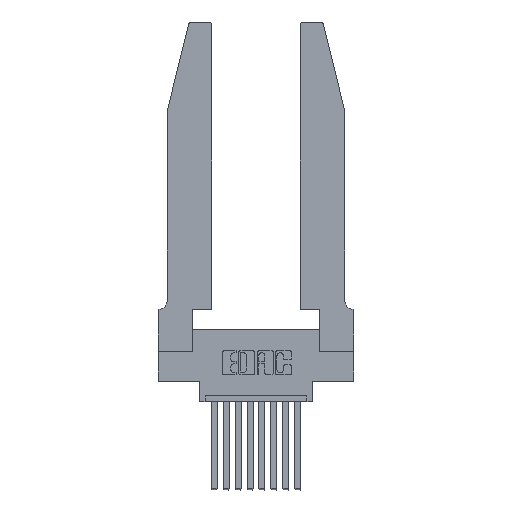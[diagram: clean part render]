
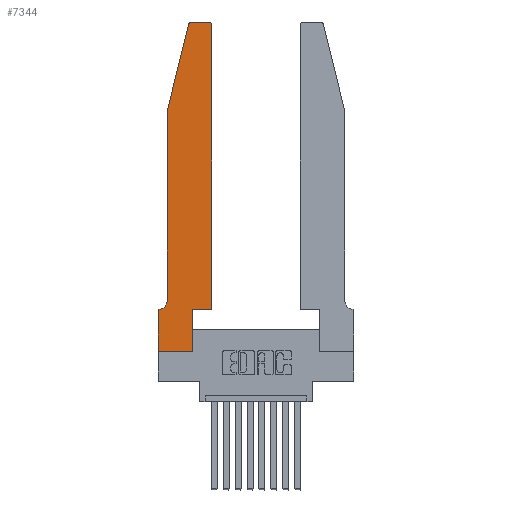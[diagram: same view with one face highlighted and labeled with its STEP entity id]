
A CAD part, top view. The second image highlights one B-rep face of the part: STEP entity #7344.
In plain terms, the highlighted planar face has unit normal (0, 0, 1).
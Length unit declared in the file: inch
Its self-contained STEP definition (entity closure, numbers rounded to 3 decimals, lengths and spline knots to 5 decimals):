
#41 = EDGE_CURVE ( 'NONE', #12247, #8929, #467, .T. ) ;
#159 = CARTESIAN_POINT ( 'NONE',  ( 0.2865, 0.35, 0.37 ) ) ;
#467 = LINE ( 'NONE', #1567, #12608 ) ;
#537 = LINE ( 'NONE', #10434, #8057 ) ;
#677 = DIRECTION ( 'NONE',  ( 0., 0., 1. ) ) ;
#807 = CARTESIAN_POINT ( 'NONE',  ( 0., 0.35, 0.37 ) ) ;
#912 = VERTEX_POINT ( 'NONE', #8366 ) ;
#1132 = VECTOR ( 'NONE', #11473, 39.37008 ) ;
#1176 = VECTOR ( 'NONE', #4415, 39.37008 ) ;
#1204 = LINE ( 'NONE', #14419, #13543 ) ;
#1209 = ORIENTED_EDGE ( 'NONE', *, *, #1664, .T. ) ;
#1481 = ORIENTED_EDGE ( 'NONE', *, *, #13996, .T. ) ;
#1500 = LINE ( 'NONE', #4461, #1132 ) ;
#1567 = CARTESIAN_POINT ( 'NONE',  ( 0.4505, 0.35, 0.37 ) ) ;
#1613 = VERTEX_POINT ( 'NONE', #807 ) ;
#1664 = EDGE_CURVE ( 'NONE', #12188, #10564, #9046, .T. ) ;
#2056 = DIRECTION ( 'NONE',  ( 0., 0., 1. ) ) ;
#2314 = DIRECTION ( 'NONE',  ( 1., 0., 0. ) ) ;
#2429 = EDGE_CURVE ( 'NONE', #1613, #5534, #3317, .T. ) ;
#2554 = LINE ( 'NONE', #5331, #10061 ) ;
#2669 = EDGE_CURVE ( 'NONE', #4311, #4338, #8298, .T. ) ;
#2743 = DIRECTION ( 'NONE',  ( 0., 1., 0. ) ) ;
#2781 = VERTEX_POINT ( 'NONE', #11555 ) ;
#3194 = EDGE_CURVE ( 'NONE', #14027, #912, #1500, .T. ) ;
#3317 = LINE ( 'NONE', #3594, #4411 ) ;
#3534 = CARTESIAN_POINT ( 'NONE',  ( 0.2605, 2.75, 0.37 ) ) ;
#3594 = CARTESIAN_POINT ( 'NONE',  ( 0., 0., 0.37 ) ) ;
#4102 = ORIENTED_EDGE ( 'NONE', *, *, #4300, .T. ) ;
#4300 = EDGE_CURVE ( 'NONE', #912, #2781, #10991, .T. ) ;
#4311 = VERTEX_POINT ( 'NONE', #12748 ) ;
#4338 = VERTEX_POINT ( 'NONE', #9152 ) ;
#4411 = VECTOR ( 'NONE', #5947, 39.37008 ) ;
#4415 = DIRECTION ( 'NONE',  ( 0., 1., 0. ) ) ;
#4461 = CARTESIAN_POINT ( 'NONE',  ( 0.0755, 2., 0.37 ) ) ;
#4563 = ORIENTED_EDGE ( 'NONE', *, *, #41, .T. ) ;
#4701 = DIRECTION ( 'NONE',  ( -1., 0., 0. ) ) ;
#4733 = CARTESIAN_POINT ( 'NONE',  ( 0., 0.35, 0.37 ) ) ;
#4869 = DIRECTION ( 'NONE',  ( -1., 0., 0. ) ) ;
#5176 = CARTESIAN_POINT ( 'NONE',  ( 0.0755, 2., 0.37 ) ) ;
#5331 = CARTESIAN_POINT ( 'NONE',  ( 0.4505, 0.35, 0.37 ) ) ;
#5497 = EDGE_CURVE ( 'NONE', #2781, #1613, #7866, .T. ) ;
#5534 = VERTEX_POINT ( 'NONE', #6351 ) ;
#5687 = DIRECTION ( 'NONE',  ( 0., 0., -1. ) ) ;
#5721 = CARTESIAN_POINT ( 'NONE',  ( 0.4505, 0.35, 0.37 ) ) ;
#5947 = DIRECTION ( 'NONE',  ( 0., -1., 0. ) ) ;
#6151 = VECTOR ( 'NONE', #4701, 39.37008 ) ;
#6347 = ORIENTED_EDGE ( 'NONE', *, *, #6669, .T. ) ;
#6351 = CARTESIAN_POINT ( 'NONE',  ( 0., 0., 0.37 ) ) ;
#6452 = AXIS2_PLACEMENT_3D ( 'NONE', #13751, #677, #8932 ) ;
#6669 = EDGE_CURVE ( 'NONE', #9208, #4311, #12627, .T. ) ;
#6671 = CARTESIAN_POINT ( 'NONE',  ( 0.4205, 2.72, 0.37 ) ) ;
#6713 = DIRECTION ( 'NONE',  ( 1., 0., 0. ) ) ;
#6739 = ORIENTED_EDGE ( 'NONE', *, *, #10433, .T. ) ;
#6947 = CARTESIAN_POINT ( 'NONE',  ( 0.2865, 0.35, 0.37 ) ) ;
#7120 = EDGE_CURVE ( 'NONE', #8929, #9208, #11308, .T. ) ;
#7344 = ADVANCED_FACE ( 'NONE', ( #13559 ), #10563, .T. ) ;
#7866 = LINE ( 'NONE', #12050, #9863 ) ;
#7882 = CARTESIAN_POINT ( 'NONE',  ( 0.0055, 0.42, 0.37 ) ) ;
#8033 = DIRECTION ( 'NONE',  ( -1., 0., 0. ) ) ;
#8057 = VECTOR ( 'NONE', #9217, 39.37008 ) ;
#8194 = EDGE_CURVE ( 'NONE', #5534, #12188, #537, .T. ) ;
#8298 = CIRCLE ( 'NONE', #6452, 0.03 ) ;
#8366 = CARTESIAN_POINT ( 'NONE',  ( 0.0755, 0.42, 0.37 ) ) ;
#8929 = VERTEX_POINT ( 'NONE', #10287 ) ;
#8932 = DIRECTION ( 'NONE',  ( 1., 0., 0. ) ) ;
#9040 = AXIS2_PLACEMENT_3D ( 'NONE', #6671, #2056, #6713 ) ;
#9046 = LINE ( 'NONE', #6947, #1176 ) ;
#9152 = CARTESIAN_POINT ( 'NONE',  ( 0.25487, 2.72718, 0.37 ) ) ;
#9208 = VERTEX_POINT ( 'NONE', #12964 ) ;
#9217 = DIRECTION ( 'NONE',  ( 1., 0., 0. ) ) ;
#9350 = AXIS2_PLACEMENT_3D ( 'NONE', #4733, #14141, #2314 ) ;
#9755 = DIRECTION ( 'NONE',  ( -0.239, -0.971, 0. ) ) ;
#9863 = VECTOR ( 'NONE', #4869, 39.37008 ) ;
#10061 = VECTOR ( 'NONE', #15079, 39.37008 ) ;
#10287 = CARTESIAN_POINT ( 'NONE',  ( 0.4505, 2.72, 0.37 ) ) ;
#10400 = EDGE_LOOP ( 'NONE', ( #6347, #11485, #1481, #10679, #4102, #15238, #10844, #11844, #1209, #6739, #4563, #12062 ) ) ;
#10433 = EDGE_CURVE ( 'NONE', #10564, #12247, #2554, .T. ) ;
#10434 = CARTESIAN_POINT ( 'NONE',  ( 0., 0., 0.37 ) ) ;
#10563 = PLANE ( 'NONE',  #9350 ) ;
#10564 = VERTEX_POINT ( 'NONE', #159 ) ;
#10679 = ORIENTED_EDGE ( 'NONE', *, *, #3194, .T. ) ;
#10844 = ORIENTED_EDGE ( 'NONE', *, *, #2429, .T. ) ;
#10991 = CIRCLE ( 'NONE', #11893, 0.07 ) ;
#11308 = CIRCLE ( 'NONE', #9040, 0.03 ) ;
#11473 = DIRECTION ( 'NONE',  ( 0., -1., 0. ) ) ;
#11485 = ORIENTED_EDGE ( 'NONE', *, *, #2669, .T. ) ;
#11555 = CARTESIAN_POINT ( 'NONE',  ( 0.0055, 0.35, 0.37 ) ) ;
#11844 = ORIENTED_EDGE ( 'NONE', *, *, #8194, .T. ) ;
#11893 = AXIS2_PLACEMENT_3D ( 'NONE', #7882, #5687, #8033 ) ;
#12050 = CARTESIAN_POINT ( 'NONE',  ( 0.0755, 0.35, 0.37 ) ) ;
#12062 = ORIENTED_EDGE ( 'NONE', *, *, #7120, .T. ) ;
#12188 = VERTEX_POINT ( 'NONE', #12265 ) ;
#12247 = VERTEX_POINT ( 'NONE', #5721 ) ;
#12265 = CARTESIAN_POINT ( 'NONE',  ( 0.2865, 0., 0.37 ) ) ;
#12608 = VECTOR ( 'NONE', #2743, 39.37008 ) ;
#12627 = LINE ( 'NONE', #3534, #6151 ) ;
#12748 = CARTESIAN_POINT ( 'NONE',  ( 0.284, 2.75, 0.37 ) ) ;
#12964 = CARTESIAN_POINT ( 'NONE',  ( 0.4205, 2.75, 0.37 ) ) ;
#13543 = VECTOR ( 'NONE', #9755, 39.37008 ) ;
#13559 = FACE_OUTER_BOUND ( 'NONE', #10400, .T. ) ;
#13751 = CARTESIAN_POINT ( 'NONE',  ( 0.284, 2.72, 0.37 ) ) ;
#13996 = EDGE_CURVE ( 'NONE', #4338, #14027, #1204, .T. ) ;
#14027 = VERTEX_POINT ( 'NONE', #5176 ) ;
#14141 = DIRECTION ( 'NONE',  ( 0., 0., 1. ) ) ;
#14419 = CARTESIAN_POINT ( 'NONE',  ( 0.0755, 2., 0.37 ) ) ;
#15079 = DIRECTION ( 'NONE',  ( 1., 0., 0. ) ) ;
#15238 = ORIENTED_EDGE ( 'NONE', *, *, #5497, .T. ) ;
